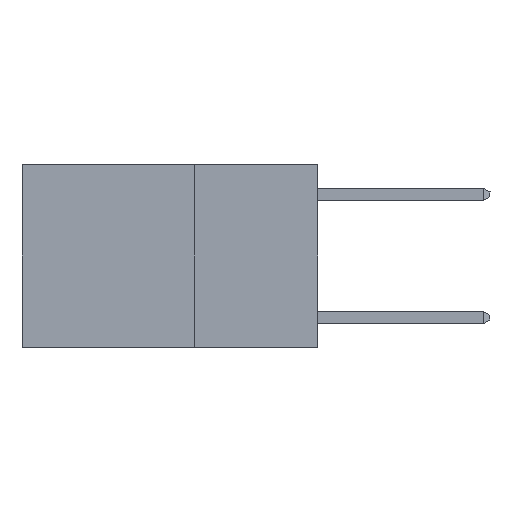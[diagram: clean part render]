
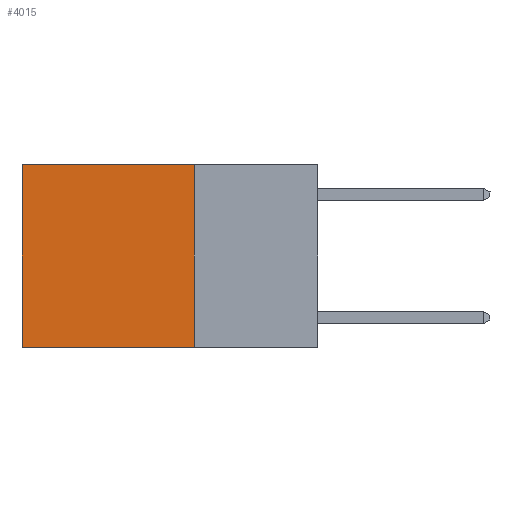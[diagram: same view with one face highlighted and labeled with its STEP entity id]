
A CAD part, left-side view. The second image highlights one B-rep face of the part: STEP entity #4015.
In plain terms, the highlighted planar face has unit normal (-1, 0, 0).
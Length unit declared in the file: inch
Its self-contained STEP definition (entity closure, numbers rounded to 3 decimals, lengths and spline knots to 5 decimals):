
#232 = VERTEX_POINT ( 'NONE', #4721 ) ;
#1255 = VECTOR ( 'NONE', #5601, 39.37008 ) ;
#1805 = EDGE_CURVE ( 'NONE', #2201, #232, #3100, .T. ) ;
#2122 = CARTESIAN_POINT ( 'NONE',  ( 0.2625, 0.25, 0. ) ) ;
#2201 = VERTEX_POINT ( 'NONE', #2484 ) ;
#2484 = CARTESIAN_POINT ( 'NONE',  ( 0.2625, 0.25, 0. ) ) ;
#2724 = CARTESIAN_POINT ( 'NONE',  ( 0.2625, 0.25, 0. ) ) ;
#2868 = VECTOR ( 'NONE', #7038, 39.37008 ) ;
#3072 = LINE ( 'NONE', #3379, #4405 ) ;
#3100 = LINE ( 'NONE', #4798, #2868 ) ;
#3181 = ORIENTED_EDGE ( 'NONE', *, *, #1805, .F. ) ;
#3308 = EDGE_CURVE ( 'NONE', #2201, #9719, #8825, .T. ) ;
#3379 = CARTESIAN_POINT ( 'NONE',  ( 0.2625, 0.25, -0.37 ) ) ;
#3454 = FACE_OUTER_BOUND ( 'NONE', #5290, .T. ) ;
#3511 = DIRECTION ( 'NONE',  ( 0., 0., -1. ) ) ;
#3587 = CARTESIAN_POINT ( 'NONE',  ( 0.2625, 0.6, -0.37 ) ) ;
#3875 = EDGE_CURVE ( 'NONE', #232, #8886, #3072, .T. ) ;
#4015 = ADVANCED_FACE ( 'NONE', ( #3454 ), #7947, .F. ) ;
#4152 = DIRECTION ( 'NONE',  ( 0., 1., 0. ) ) ;
#4401 = ORIENTED_EDGE ( 'NONE', *, *, #3308, .T. ) ;
#4405 = VECTOR ( 'NONE', #4152, 39.37008 ) ;
#4721 = CARTESIAN_POINT ( 'NONE',  ( 0.2625, 0.25, -0.37 ) ) ;
#4798 = CARTESIAN_POINT ( 'NONE',  ( 0.2625, 0.25, 0. ) ) ;
#5199 = CARTESIAN_POINT ( 'NONE',  ( 0.2625, 0.6, 0. ) ) ;
#5290 = EDGE_LOOP ( 'NONE', ( #7335, #8658, #3181, #4401 ) ) ;
#5506 = AXIS2_PLACEMENT_3D ( 'NONE', #2724, #7980, #3511 ) ;
#5601 = DIRECTION ( 'NONE',  ( 0., 0., -1. ) ) ;
#7038 = DIRECTION ( 'NONE',  ( 0., 0., -1. ) ) ;
#7103 = VECTOR ( 'NONE', #7789, 39.37008 ) ;
#7335 = ORIENTED_EDGE ( 'NONE', *, *, #8566, .T. ) ;
#7344 = LINE ( 'NONE', #8531, #1255 ) ;
#7789 = DIRECTION ( 'NONE',  ( 0., 1., 0. ) ) ;
#7947 = PLANE ( 'NONE',  #5506 ) ;
#7980 = DIRECTION ( 'NONE',  ( 1., 0., 0. ) ) ;
#8531 = CARTESIAN_POINT ( 'NONE',  ( 0.2625, 0.6, 0. ) ) ;
#8566 = EDGE_CURVE ( 'NONE', #9719, #8886, #7344, .T. ) ;
#8658 = ORIENTED_EDGE ( 'NONE', *, *, #3875, .F. ) ;
#8825 = LINE ( 'NONE', #2122, #7103 ) ;
#8886 = VERTEX_POINT ( 'NONE', #3587 ) ;
#9719 = VERTEX_POINT ( 'NONE', #5199 ) ;
